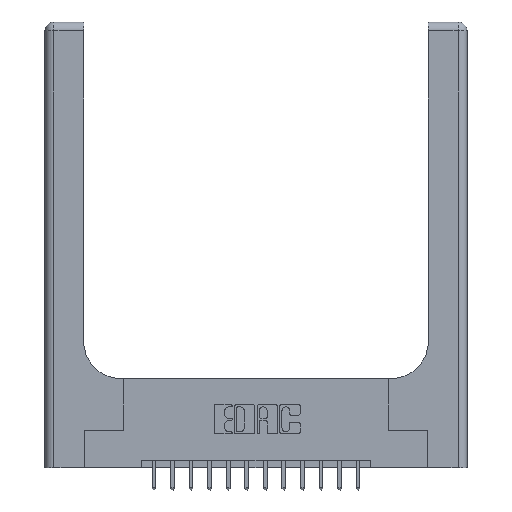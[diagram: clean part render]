
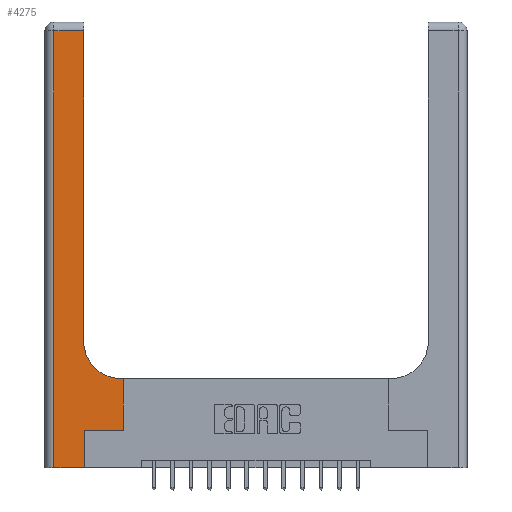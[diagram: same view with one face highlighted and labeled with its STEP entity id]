
A CAD part, top view. The second image highlights one B-rep face of the part: STEP entity #4275.
In plain terms, the highlighted planar face has unit normal (0, 0, 1).
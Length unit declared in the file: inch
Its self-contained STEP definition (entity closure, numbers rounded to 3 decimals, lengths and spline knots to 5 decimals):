
#145 = VECTOR ( 'NONE', #3468, 39.37008 ) ;
#579 = CARTESIAN_POINT ( 'NONE',  ( 0.26, 0.85, 0.37 ) ) ;
#774 = ORIENTED_EDGE ( 'NONE', *, *, #2442, .T. ) ;
#801 = CARTESIAN_POINT ( 'NONE',  ( 0.26, 0.6, 0.37 ) ) ;
#903 = DIRECTION ( 'NONE',  ( -1., 0., 0. ) ) ;
#1041 = LINE ( 'NONE', #7611, #8300 ) ;
#1267 = VERTEX_POINT ( 'NONE', #2639 ) ;
#1343 = DIRECTION ( 'NONE',  ( 1., 0., 0. ) ) ;
#1606 = CARTESIAN_POINT ( 'NONE',  ( 0.265, 0.25, 0.37 ) ) ;
#1675 = DIRECTION ( 'NONE',  ( 0., 1., 0. ) ) ;
#1790 = VECTOR ( 'NONE', #7025, 39.37008 ) ;
#2247 = ORIENTED_EDGE ( 'NONE', *, *, #2673, .T. ) ;
#2414 = FACE_OUTER_BOUND ( 'NONE', #4005, .T. ) ;
#2442 = EDGE_CURVE ( 'NONE', #1267, #13454, #1041, .T. ) ;
#2639 = CARTESIAN_POINT ( 'NONE',  ( 0.06, 2.94, 0.37 ) ) ;
#2673 = EDGE_CURVE ( 'NONE', #14919, #16738, #6717, .T. ) ;
#2767 = LINE ( 'NONE', #15391, #9100 ) ;
#2965 = VERTEX_POINT ( 'NONE', #10158 ) ;
#3468 = DIRECTION ( 'NONE',  ( -1., 0., 0. ) ) ;
#4005 = EDGE_LOOP ( 'NONE', ( #2247, #6969, #774, #11998, #7333, #11000, #4635, #5335, #11437 ) ) ;
#4224 = DIRECTION ( 'NONE',  ( 0., 1., 0. ) ) ;
#4275 = ADVANCED_FACE ( 'NONE', ( #2414 ), #15698, .F. ) ;
#4354 = LINE ( 'NONE', #13999, #12668 ) ;
#4544 = DIRECTION ( 'NONE',  ( -1., 0., 0. ) ) ;
#4605 = CARTESIAN_POINT ( 'NONE',  ( 0.51, 0.85, 0.37 ) ) ;
#4635 = ORIENTED_EDGE ( 'NONE', *, *, #7529, .T. ) ;
#5335 = ORIENTED_EDGE ( 'NONE', *, *, #8130, .T. ) ;
#5883 = CARTESIAN_POINT ( 'NONE',  ( 0., 2.94, 0.37 ) ) ;
#6061 = AXIS2_PLACEMENT_3D ( 'NONE', #4605, #8428, #13898 ) ;
#6405 = DIRECTION ( 'NONE',  ( 0., 0., -1. ) ) ;
#6717 = LINE ( 'NONE', #16368, #15598 ) ;
#6772 = CARTESIAN_POINT ( 'NONE',  ( 0.26, 2.94, 0.37 ) ) ;
#6959 = VERTEX_POINT ( 'NONE', #17317 ) ;
#6969 = ORIENTED_EDGE ( 'NONE', *, *, #12529, .T. ) ;
#6987 = EDGE_CURVE ( 'NONE', #2965, #6959, #9781, .T. ) ;
#7025 = DIRECTION ( 'NONE',  ( 1., 0., 0. ) ) ;
#7270 = LINE ( 'NONE', #10008, #10588 ) ;
#7333 = ORIENTED_EDGE ( 'NONE', *, *, #12930, .T. ) ;
#7508 = EDGE_CURVE ( 'NONE', #7774, #14919, #13698, .T. ) ;
#7529 = EDGE_CURVE ( 'NONE', #6959, #16441, #7270, .T. ) ;
#7611 = CARTESIAN_POINT ( 'NONE',  ( 0.06, 3., 0.37 ) ) ;
#7774 = VERTEX_POINT ( 'NONE', #15634 ) ;
#8130 = EDGE_CURVE ( 'NONE', #16441, #7774, #13028, .T. ) ;
#8300 = VECTOR ( 'NONE', #14413, 39.37008 ) ;
#8428 = DIRECTION ( 'NONE',  ( 0., 0., -1. ) ) ;
#8461 = VECTOR ( 'NONE', #4544, 39.37008 ) ;
#9100 = VECTOR ( 'NONE', #1343, 39.37008 ) ;
#9516 = VERTEX_POINT ( 'NONE', #13834 ) ;
#9781 = LINE ( 'NONE', #1606, #1790 ) ;
#9933 = DIRECTION ( 'NONE',  ( 0., 1., 0. ) ) ;
#10008 = CARTESIAN_POINT ( 'NONE',  ( 0.528, 0.25, 0.37 ) ) ;
#10158 = CARTESIAN_POINT ( 'NONE',  ( 0.265, 0.25, 0.37 ) ) ;
#10588 = VECTOR ( 'NONE', #1675, 39.37008 ) ;
#11000 = ORIENTED_EDGE ( 'NONE', *, *, #6987, .T. ) ;
#11280 = LINE ( 'NONE', #5883, #8461 ) ;
#11437 = ORIENTED_EDGE ( 'NONE', *, *, #7508, .T. ) ;
#11998 = ORIENTED_EDGE ( 'NONE', *, *, #17272, .T. ) ;
#12529 = EDGE_CURVE ( 'NONE', #16738, #1267, #11280, .T. ) ;
#12668 = VECTOR ( 'NONE', #9933, 39.37008 ) ;
#12930 = EDGE_CURVE ( 'NONE', #9516, #2965, #4354, .T. ) ;
#13028 = LINE ( 'NONE', #801, #145 ) ;
#13454 = VERTEX_POINT ( 'NONE', #14233 ) ;
#13698 = CIRCLE ( 'NONE', #6061, 0.25 ) ;
#13834 = CARTESIAN_POINT ( 'NONE',  ( 0.265, 0., 0.37 ) ) ;
#13898 = DIRECTION ( 'NONE',  ( 1., 0., 0. ) ) ;
#13999 = CARTESIAN_POINT ( 'NONE',  ( 0.265, 0., 0.37 ) ) ;
#14233 = CARTESIAN_POINT ( 'NONE',  ( 0.06, 0., 0.37 ) ) ;
#14413 = DIRECTION ( 'NONE',  ( 0., -1., 0. ) ) ;
#14919 = VERTEX_POINT ( 'NONE', #579 ) ;
#15193 = CARTESIAN_POINT ( 'NONE',  ( 0.528, 0.6, 0.37 ) ) ;
#15391 = CARTESIAN_POINT ( 'NONE',  ( 0., 0., 0.37 ) ) ;
#15598 = VECTOR ( 'NONE', #4224, 39.37008 ) ;
#15605 = CARTESIAN_POINT ( 'NONE',  ( 0., 3., 0.37 ) ) ;
#15634 = CARTESIAN_POINT ( 'NONE',  ( 0.51, 0.6, 0.37 ) ) ;
#15698 = PLANE ( 'NONE',  #16220 ) ;
#16220 = AXIS2_PLACEMENT_3D ( 'NONE', #15605, #6405, #903 ) ;
#16368 = CARTESIAN_POINT ( 'NONE',  ( 0.26, 3., 0.37 ) ) ;
#16441 = VERTEX_POINT ( 'NONE', #15193 ) ;
#16738 = VERTEX_POINT ( 'NONE', #6772 ) ;
#17272 = EDGE_CURVE ( 'NONE', #13454, #9516, #2767, .T. ) ;
#17317 = CARTESIAN_POINT ( 'NONE',  ( 0.528, 0.25, 0.37 ) ) ;
